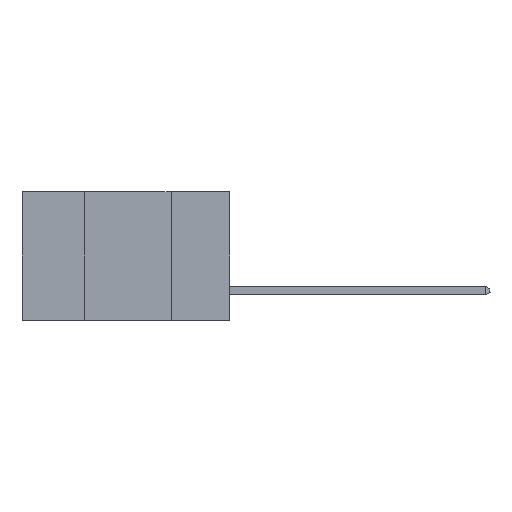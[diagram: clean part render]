
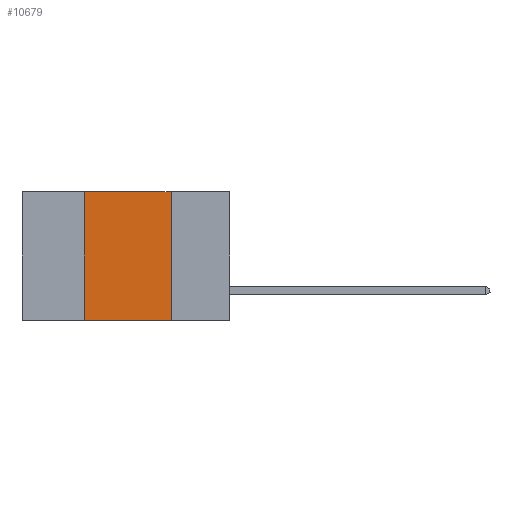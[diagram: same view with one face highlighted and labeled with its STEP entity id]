
A CAD part, left-side view. The second image highlights one B-rep face of the part: STEP entity #10679.
In plain terms, the highlighted planar face has unit normal (-1, 0, 0).
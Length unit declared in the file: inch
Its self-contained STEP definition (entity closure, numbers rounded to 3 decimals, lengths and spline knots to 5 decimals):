
#238 = VECTOR ( 'NONE', #1723, 39.37008 ) ;
#529 = EDGE_CURVE ( 'NONE', #4767, #849, #7337, .T. ) ;
#679 = LINE ( 'NONE', #10797, #6821 ) ;
#818 = PLANE ( 'NONE',  #6741 ) ;
#849 = VERTEX_POINT ( 'NONE', #12152 ) ;
#1207 = DIRECTION ( 'NONE',  ( 0., 0., 1. ) ) ;
#1418 = LINE ( 'NONE', #10716, #4862 ) ;
#1723 = DIRECTION ( 'NONE',  ( 0., 0., -1. ) ) ;
#2032 = DIRECTION ( 'NONE',  ( 0., -1., 0. ) ) ;
#2211 = ORIENTED_EDGE ( 'NONE', *, *, #4692, .F. ) ;
#2342 = EDGE_CURVE ( 'NONE', #3314, #11239, #679, .T. ) ;
#3314 = VERTEX_POINT ( 'NONE', #4249 ) ;
#3431 = ORIENTED_EDGE ( 'NONE', *, *, #7662, .F. ) ;
#3648 = CARTESIAN_POINT ( 'NONE',  ( 0., 0.17, 0. ) ) ;
#4249 = CARTESIAN_POINT ( 'NONE',  ( 0., 0.42, -0.37 ) ) ;
#4692 = EDGE_CURVE ( 'NONE', #849, #11239, #5199, .T. ) ;
#4767 = VERTEX_POINT ( 'NONE', #11351 ) ;
#4862 = VECTOR ( 'NONE', #1207, 39.37008 ) ;
#5199 = LINE ( 'NONE', #3648, #238 ) ;
#5815 = CARTESIAN_POINT ( 'NONE',  ( 0., 0.17, -0.37 ) ) ;
#6133 = ORIENTED_EDGE ( 'NONE', *, *, #529, .F. ) ;
#6741 = AXIS2_PLACEMENT_3D ( 'NONE', #11261, #7520, #11298 ) ;
#6821 = VECTOR ( 'NONE', #12236, 39.37008 ) ;
#7337 = LINE ( 'NONE', #8666, #9854 ) ;
#7520 = DIRECTION ( 'NONE',  ( 1., 0., 0. ) ) ;
#7662 = EDGE_CURVE ( 'NONE', #3314, #4767, #1418, .T. ) ;
#8417 = ORIENTED_EDGE ( 'NONE', *, *, #2342, .T. ) ;
#8666 = CARTESIAN_POINT ( 'NONE',  ( 0., 0.6, 0. ) ) ;
#9854 = VECTOR ( 'NONE', #2032, 39.37008 ) ;
#10321 = EDGE_LOOP ( 'NONE', ( #2211, #6133, #3431, #8417 ) ) ;
#10679 = ADVANCED_FACE ( 'NONE', ( #12111 ), #818, .F. ) ;
#10716 = CARTESIAN_POINT ( 'NONE',  ( 0., 0.42, 0. ) ) ;
#10797 = CARTESIAN_POINT ( 'NONE',  ( 0., 0.6, -0.37 ) ) ;
#11239 = VERTEX_POINT ( 'NONE', #5815 ) ;
#11261 = CARTESIAN_POINT ( 'NONE',  ( 0., 0.6, 0. ) ) ;
#11298 = DIRECTION ( 'NONE',  ( 0., 0., -1. ) ) ;
#11351 = CARTESIAN_POINT ( 'NONE',  ( 0., 0.42, 0. ) ) ;
#12111 = FACE_OUTER_BOUND ( 'NONE', #10321, .T. ) ;
#12152 = CARTESIAN_POINT ( 'NONE',  ( 0., 0.17, 0. ) ) ;
#12236 = DIRECTION ( 'NONE',  ( 0., -1., 0. ) ) ;
